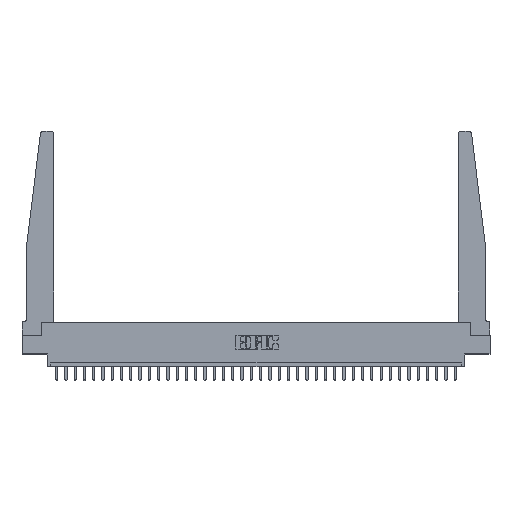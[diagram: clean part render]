
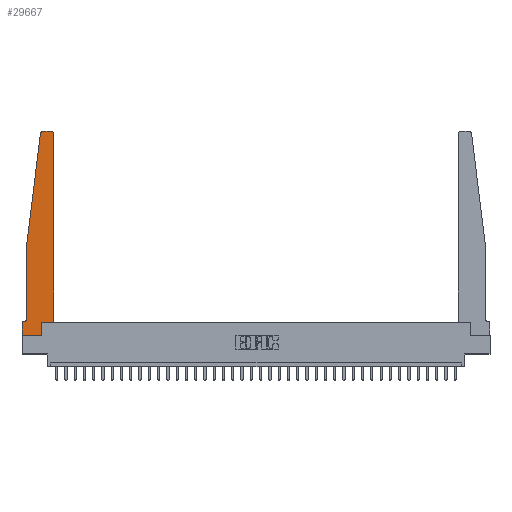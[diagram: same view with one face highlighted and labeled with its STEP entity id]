
A CAD part, top view. The second image highlights one B-rep face of the part: STEP entity #29667.
In plain terms, the highlighted planar face has unit normal (0, 0, 1).
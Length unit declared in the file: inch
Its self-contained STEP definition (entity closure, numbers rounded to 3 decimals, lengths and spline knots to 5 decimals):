
#60 = EDGE_CURVE ( 'NONE', #7074, #6691, #5284, .T. ) ;
#116 = EDGE_CURVE ( 'NONE', #20684, #26897, #18928, .T. ) ;
#617 = EDGE_CURVE ( 'NONE', #8841, #20684, #4130, .T. ) ;
#859 = VECTOR ( 'NONE', #10340, 39.37008 ) ;
#1016 = DIRECTION ( 'NONE',  ( 1., 0., 0. ) ) ;
#1942 = LINE ( 'NONE', #16746, #11565 ) ;
#2204 = VERTEX_POINT ( 'NONE', #18268 ) ;
#2800 = ORIENTED_EDGE ( 'NONE', *, *, #23981, .T. ) ;
#2825 = DIRECTION ( 'NONE',  ( 0., 0., 1. ) ) ;
#3397 = LINE ( 'NONE', #21308, #31010 ) ;
#3526 = VERTEX_POINT ( 'NONE', #11486 ) ;
#3696 = VECTOR ( 'NONE', #27827, 39.37008 ) ;
#3849 = DIRECTION ( 'NONE',  ( 0., 0., 1. ) ) ;
#3985 = CARTESIAN_POINT ( 'NONE',  ( 0.065, 1.25, 0.37 ) ) ;
#4130 = LINE ( 'NONE', #31902, #7972 ) ;
#4734 = AXIS2_PLACEMENT_3D ( 'NONE', #23364, #2825, #1016 ) ;
#4892 = ORIENTED_EDGE ( 'NONE', *, *, #617, .T. ) ;
#5058 = CARTESIAN_POINT ( 'NONE',  ( 0., 0., 0.37 ) ) ;
#5284 = LINE ( 'NONE', #28466, #3696 ) ;
#5294 = EDGE_CURVE ( 'NONE', #26897, #28518, #18025, .T. ) ;
#5508 = DIRECTION ( 'NONE',  ( -1., 0., 0. ) ) ;
#6064 = VERTEX_POINT ( 'NONE', #16399 ) ;
#6481 = CARTESIAN_POINT ( 'NONE',  ( 0.2605, 0., 0.37 ) ) ;
#6691 = VERTEX_POINT ( 'NONE', #11735 ) ;
#6867 = VECTOR ( 'NONE', #5508, 39.37008 ) ;
#7074 = VERTEX_POINT ( 'NONE', #16164 ) ;
#7241 = DIRECTION ( 'NONE',  ( 1., 0., 0. ) ) ;
#7386 = ORIENTED_EDGE ( 'NONE', *, *, #5294, .T. ) ;
#7972 = VECTOR ( 'NONE', #9518, 39.37008 ) ;
#8459 = CARTESIAN_POINT ( 'NONE',  ( 0.015, 0.2375, 0.37 ) ) ;
#8495 = EDGE_CURVE ( 'NONE', #28518, #2204, #19041, .T. ) ;
#8841 = VERTEX_POINT ( 'NONE', #32441 ) ;
#9518 = DIRECTION ( 'NONE',  ( 0., 1., 0. ) ) ;
#9955 = EDGE_CURVE ( 'NONE', #6064, #29612, #31168, .T. ) ;
#10067 = AXIS2_PLACEMENT_3D ( 'NONE', #26531, #3849, #26211 ) ;
#10340 = DIRECTION ( 'NONE',  ( 0., -1., 0. ) ) ;
#10359 = CARTESIAN_POINT ( 'NONE',  ( 0.425, 0.18, 0.37 ) ) ;
#10445 = DIRECTION ( 'NONE',  ( -1., 0., 0. ) ) ;
#11486 = CARTESIAN_POINT ( 'NONE',  ( 0.2605, 0.18, 0.37 ) ) ;
#11565 = VECTOR ( 'NONE', #12103, 39.37008 ) ;
#11710 = ORIENTED_EDGE ( 'NONE', *, *, #116, .T. ) ;
#11735 = CARTESIAN_POINT ( 'NONE',  ( 0., 0., 0.37 ) ) ;
#12010 = CARTESIAN_POINT ( 'NONE',  ( 0.27653, 2.72, 0.37 ) ) ;
#12103 = DIRECTION ( 'NONE',  ( 0., 1., 0. ) ) ;
#12112 = ORIENTED_EDGE ( 'NONE', *, *, #60, .T. ) ;
#12888 = CARTESIAN_POINT ( 'NONE',  ( 0.425, 2.72, 0.37 ) ) ;
#13459 = CARTESIAN_POINT ( 'NONE',  ( 0.065, 1.25, 0.37 ) ) ;
#13592 = VERTEX_POINT ( 'NONE', #3985 ) ;
#14622 = VECTOR ( 'NONE', #29940, 39.37008 ) ;
#15274 = DIRECTION ( 'NONE',  ( -1., 0., 0. ) ) ;
#15438 = LINE ( 'NONE', #30233, #28952 ) ;
#16014 = CARTESIAN_POINT ( 'NONE',  ( 0.27653, 2.75, 0.37 ) ) ;
#16164 = CARTESIAN_POINT ( 'NONE',  ( 0., 0.1875, 0.37 ) ) ;
#16399 = CARTESIAN_POINT ( 'NONE',  ( 0.065, 0.2375, 0.37 ) ) ;
#16444 = ORIENTED_EDGE ( 'NONE', *, *, #9955, .T. ) ;
#16746 = CARTESIAN_POINT ( 'NONE',  ( 0.2605, 0.18, 0.37 ) ) ;
#17102 = ORIENTED_EDGE ( 'NONE', *, *, #27126, .T. ) ;
#17376 = ORIENTED_EDGE ( 'NONE', *, *, #27416, .T. ) ;
#18025 = LINE ( 'NONE', #28045, #6867 ) ;
#18268 = CARTESIAN_POINT ( 'NONE',  ( 0.24675, 2.72367, 0.37 ) ) ;
#18270 = ORIENTED_EDGE ( 'NONE', *, *, #8495, .T. ) ;
#18682 = DIRECTION ( 'NONE',  ( -0.122, -0.992, 0. ) ) ;
#18928 = CIRCLE ( 'NONE', #4734, 0.03 ) ;
#19041 = CIRCLE ( 'NONE', #23778, 0.03 ) ;
#19259 = CARTESIAN_POINT ( 'NONE',  ( 0.395, 2.75, 0.37 ) ) ;
#19288 = EDGE_CURVE ( 'NONE', #13592, #6064, #25817, .T. ) ;
#19311 = FACE_OUTER_BOUND ( 'NONE', #28042, .T. ) ;
#20205 = DIRECTION ( 'NONE',  ( 1., 0., 0. ) ) ;
#20225 = ORIENTED_EDGE ( 'NONE', *, *, #27666, .T. ) ;
#20684 = VERTEX_POINT ( 'NONE', #12888 ) ;
#21194 = AXIS2_PLACEMENT_3D ( 'NONE', #8459, #27901, #10445 ) ;
#21308 = CARTESIAN_POINT ( 'NONE',  ( 0.065, 1.25, 0.37 ) ) ;
#22209 = VERTEX_POINT ( 'NONE', #6481 ) ;
#22707 = LINE ( 'NONE', #10359, #14622 ) ;
#23364 = CARTESIAN_POINT ( 'NONE',  ( 0.395, 2.72, 0.37 ) ) ;
#23778 = AXIS2_PLACEMENT_3D ( 'NONE', #12010, #24524, #7241 ) ;
#23981 = EDGE_CURVE ( 'NONE', #3526, #8841, #22707, .T. ) ;
#24334 = EDGE_CURVE ( 'NONE', #6691, #22209, #27594, .T. ) ;
#24524 = DIRECTION ( 'NONE',  ( 0., 0., 1. ) ) ;
#24622 = VECTOR ( 'NONE', #20205, 39.37008 ) ;
#25817 = LINE ( 'NONE', #13459, #859 ) ;
#26211 = DIRECTION ( 'NONE',  ( 1., 0., 0. ) ) ;
#26531 = CARTESIAN_POINT ( 'NONE',  ( 0., 0.1875, 0.37 ) ) ;
#26897 = VERTEX_POINT ( 'NONE', #19259 ) ;
#27126 = EDGE_CURVE ( 'NONE', #29612, #7074, #15438, .T. ) ;
#27416 = EDGE_CURVE ( 'NONE', #22209, #3526, #1942, .T. ) ;
#27594 = LINE ( 'NONE', #5058, #24622 ) ;
#27666 = EDGE_CURVE ( 'NONE', #2204, #13592, #3397, .T. ) ;
#27827 = DIRECTION ( 'NONE',  ( 0., -1., 0. ) ) ;
#27901 = DIRECTION ( 'NONE',  ( 0., 0., -1. ) ) ;
#28042 = EDGE_LOOP ( 'NONE', ( #7386, #18270, #20225, #28910, #16444, #17102, #12112, #28578, #17376, #2800, #4892, #11710 ) ) ;
#28045 = CARTESIAN_POINT ( 'NONE',  ( 0.25, 2.75, 0.37 ) ) ;
#28466 = CARTESIAN_POINT ( 'NONE',  ( 0., 0., 0.37 ) ) ;
#28518 = VERTEX_POINT ( 'NONE', #16014 ) ;
#28578 = ORIENTED_EDGE ( 'NONE', *, *, #24334, .T. ) ;
#28910 = ORIENTED_EDGE ( 'NONE', *, *, #19288, .T. ) ;
#28952 = VECTOR ( 'NONE', #15274, 39.37008 ) ;
#29612 = VERTEX_POINT ( 'NONE', #30041 ) ;
#29667 = ADVANCED_FACE ( 'NONE', ( #19311 ), #31620, .T. ) ;
#29940 = DIRECTION ( 'NONE',  ( 1., 0., 0. ) ) ;
#30041 = CARTESIAN_POINT ( 'NONE',  ( 0.015, 0.1875, 0.37 ) ) ;
#30233 = CARTESIAN_POINT ( 'NONE',  ( 0.065, 0.1875, 0.37 ) ) ;
#31010 = VECTOR ( 'NONE', #18682, 39.37008 ) ;
#31168 = CIRCLE ( 'NONE', #21194, 0.05 ) ;
#31620 = PLANE ( 'NONE',  #10067 ) ;
#31902 = CARTESIAN_POINT ( 'NONE',  ( 0.425, 0.18, 0.37 ) ) ;
#32441 = CARTESIAN_POINT ( 'NONE',  ( 0.425, 0.18, 0.37 ) ) ;
